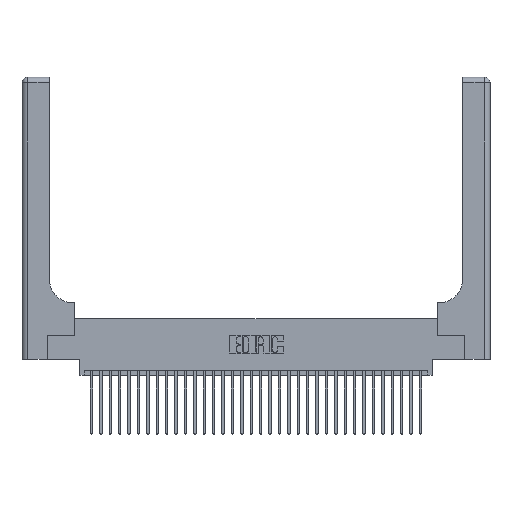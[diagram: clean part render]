
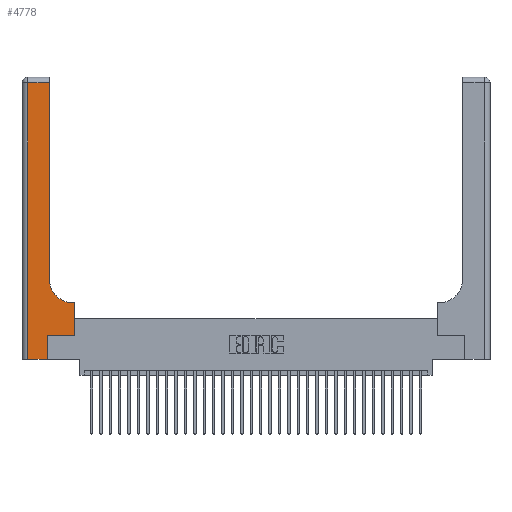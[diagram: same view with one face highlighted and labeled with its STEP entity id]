
A CAD part, top view. The second image highlights one B-rep face of the part: STEP entity #4778.
In plain terms, the highlighted planar face has unit normal (0, 0, 1).
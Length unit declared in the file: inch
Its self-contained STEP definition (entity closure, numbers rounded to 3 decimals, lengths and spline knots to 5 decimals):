
#27 = EDGE_CURVE ( 'NONE', #27619, #28350, #18687, .T. ) ;
#832 = ORIENTED_EDGE ( 'NONE', *, *, #7603, .T. ) ;
#1005 = AXIS2_PLACEMENT_3D ( 'NONE', #29059, #13326, #31732 ) ;
#2517 = ORIENTED_EDGE ( 'NONE', *, *, #27, .T. ) ;
#3674 = VERTEX_POINT ( 'NONE', #25708 ) ;
#4240 = VECTOR ( 'NONE', #19103, 39.37008 ) ;
#4436 = VECTOR ( 'NONE', #16363, 39.37008 ) ;
#4778 = ADVANCED_FACE ( 'NONE', ( #20397 ), #16590, .F. ) ;
#5913 = ORIENTED_EDGE ( 'NONE', *, *, #30246, .T. ) ;
#6601 = VERTEX_POINT ( 'NONE', #25094 ) ;
#7048 = EDGE_CURVE ( 'NONE', #28350, #7442, #11599, .T. ) ;
#7442 = VERTEX_POINT ( 'NONE', #25511 ) ;
#7491 = CARTESIAN_POINT ( 'NONE',  ( 0.269, 0., 0.37 ) ) ;
#7603 = EDGE_CURVE ( 'NONE', #3674, #17511, #9930, .T. ) ;
#7812 = EDGE_CURVE ( 'NONE', #17511, #27619, #24346, .T. ) ;
#8691 = DIRECTION ( 'NONE',  ( 0., 0., -1. ) ) ;
#9032 = VERTEX_POINT ( 'NONE', #22319 ) ;
#9595 = DIRECTION ( 'NONE',  ( 0., -1., 0. ) ) ;
#9862 = VECTOR ( 'NONE', #14426, 39.37008 ) ;
#9930 = LINE ( 'NONE', #29874, #24773 ) ;
#9994 = LINE ( 'NONE', #29517, #29363 ) ;
#10390 = DIRECTION ( 'NONE',  ( 0., 1., 0. ) ) ;
#11502 = CIRCLE ( 'NONE', #1005, 0.25 ) ;
#11599 = LINE ( 'NONE', #18880, #4436 ) ;
#12015 = EDGE_CURVE ( 'NONE', #9032, #14812, #23856, .T. ) ;
#13095 = LINE ( 'NONE', #16479, #4240 ) ;
#13326 = DIRECTION ( 'NONE',  ( 0., 0., -1. ) ) ;
#13344 = VECTOR ( 'NONE', #34070, 39.37008 ) ;
#14141 = DIRECTION ( 'NONE',  ( -1., 0., 0. ) ) ;
#14426 = DIRECTION ( 'NONE',  ( 0., 1., 0. ) ) ;
#14812 = VERTEX_POINT ( 'NONE', #31518 ) ;
#15129 = ORIENTED_EDGE ( 'NONE', *, *, #7812, .T. ) ;
#15535 = EDGE_CURVE ( 'NONE', #6601, #3674, #16256, .T. ) ;
#15741 = CARTESIAN_POINT ( 'NONE',  ( 0.2915, 3., 0.37 ) ) ;
#16256 = LINE ( 'NONE', #15741, #29384 ) ;
#16363 = DIRECTION ( 'NONE',  ( 0., 1., 0. ) ) ;
#16479 = CARTESIAN_POINT ( 'NONE',  ( 0.269, 0.25, 0.37 ) ) ;
#16590 = PLANE ( 'NONE',  #31795 ) ;
#17074 = CARTESIAN_POINT ( 'NONE',  ( 0.5585, 0.25, 0.37 ) ) ;
#17511 = VERTEX_POINT ( 'NONE', #24452 ) ;
#18292 = CARTESIAN_POINT ( 'NONE',  ( 0.5415, 0.6, 0.37 ) ) ;
#18411 = ORIENTED_EDGE ( 'NONE', *, *, #12015, .T. ) ;
#18687 = LINE ( 'NONE', #34139, #13344 ) ;
#18880 = CARTESIAN_POINT ( 'NONE',  ( 0.269, 0., 0.37 ) ) ;
#19103 = DIRECTION ( 'NONE',  ( 1., 0., 0. ) ) ;
#19242 = ORIENTED_EDGE ( 'NONE', *, *, #22919, .T. ) ;
#20128 = EDGE_CURVE ( 'NONE', #7442, #9032, #13095, .T. ) ;
#20397 = FACE_OUTER_BOUND ( 'NONE', #28444, .T. ) ;
#21275 = ORIENTED_EDGE ( 'NONE', *, *, #15535, .T. ) ;
#22319 = CARTESIAN_POINT ( 'NONE',  ( 0.5585, 0.25, 0.37 ) ) ;
#22919 = EDGE_CURVE ( 'NONE', #14812, #34091, #9994, .T. ) ;
#23856 = LINE ( 'NONE', #17074, #9862 ) ;
#24346 = LINE ( 'NONE', #25370, #31351 ) ;
#24452 = CARTESIAN_POINT ( 'NONE',  ( 0.06, 2.94, 0.37 ) ) ;
#24499 = CARTESIAN_POINT ( 'NONE',  ( 0., 3., 0.37 ) ) ;
#24576 = ORIENTED_EDGE ( 'NONE', *, *, #7048, .T. ) ;
#24773 = VECTOR ( 'NONE', #14141, 39.37008 ) ;
#25094 = CARTESIAN_POINT ( 'NONE',  ( 0.2915, 0.85, 0.37 ) ) ;
#25370 = CARTESIAN_POINT ( 'NONE',  ( 0.06, 3., 0.37 ) ) ;
#25511 = CARTESIAN_POINT ( 'NONE',  ( 0.269, 0.25, 0.37 ) ) ;
#25708 = CARTESIAN_POINT ( 'NONE',  ( 0.2915, 2.94, 0.37 ) ) ;
#27140 = DIRECTION ( 'NONE',  ( -1., 0., 0. ) ) ;
#27619 = VERTEX_POINT ( 'NONE', #30996 ) ;
#28350 = VERTEX_POINT ( 'NONE', #7491 ) ;
#28444 = EDGE_LOOP ( 'NONE', ( #21275, #832, #15129, #2517, #24576, #31573, #18411, #19242, #5913 ) ) ;
#29059 = CARTESIAN_POINT ( 'NONE',  ( 0.5415, 0.85, 0.37 ) ) ;
#29363 = VECTOR ( 'NONE', #32176, 39.37008 ) ;
#29384 = VECTOR ( 'NONE', #10390, 39.37008 ) ;
#29517 = CARTESIAN_POINT ( 'NONE',  ( 0.2915, 0.6, 0.37 ) ) ;
#29874 = CARTESIAN_POINT ( 'NONE',  ( 0., 2.94, 0.37 ) ) ;
#30246 = EDGE_CURVE ( 'NONE', #34091, #6601, #11502, .T. ) ;
#30996 = CARTESIAN_POINT ( 'NONE',  ( 0.06, 0., 0.37 ) ) ;
#31351 = VECTOR ( 'NONE', #9595, 39.37008 ) ;
#31518 = CARTESIAN_POINT ( 'NONE',  ( 0.5585, 0.6, 0.37 ) ) ;
#31573 = ORIENTED_EDGE ( 'NONE', *, *, #20128, .T. ) ;
#31732 = DIRECTION ( 'NONE',  ( 1., 0., 0. ) ) ;
#31795 = AXIS2_PLACEMENT_3D ( 'NONE', #24499, #8691, #27140 ) ;
#32176 = DIRECTION ( 'NONE',  ( -1., 0., 0. ) ) ;
#34070 = DIRECTION ( 'NONE',  ( 1., 0., 0. ) ) ;
#34091 = VERTEX_POINT ( 'NONE', #18292 ) ;
#34139 = CARTESIAN_POINT ( 'NONE',  ( 0., 0., 0.37 ) ) ;
